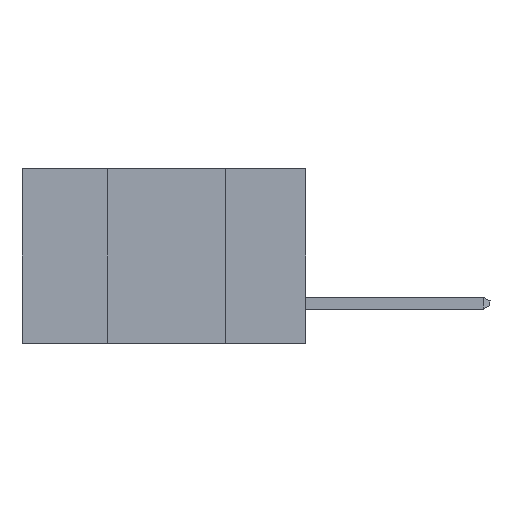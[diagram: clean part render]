
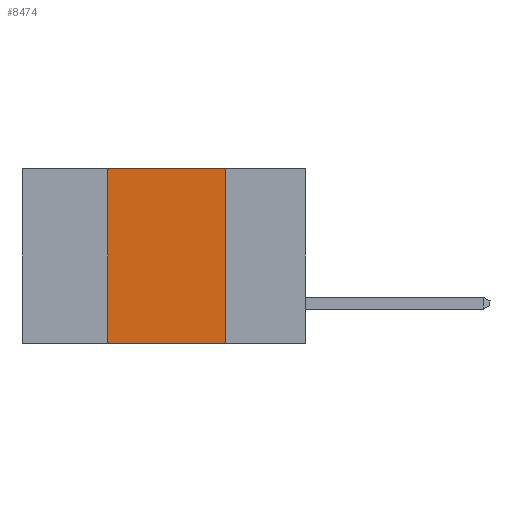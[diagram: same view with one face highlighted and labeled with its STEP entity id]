
A CAD part, left-side view. The second image highlights one B-rep face of the part: STEP entity #8474.
In plain terms, the highlighted planar face has unit normal (-1, 0, 0).
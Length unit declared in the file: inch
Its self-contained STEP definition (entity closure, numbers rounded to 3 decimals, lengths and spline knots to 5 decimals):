
#696 = CARTESIAN_POINT ( 'NONE',  ( 0., 0.42, -0.37 ) ) ;
#1284 = DIRECTION ( 'NONE',  ( 0., 0., -1. ) ) ;
#1611 = CARTESIAN_POINT ( 'NONE',  ( 0., 0.17, 0. ) ) ;
#1763 = VERTEX_POINT ( 'NONE', #1611 ) ;
#1956 = ORIENTED_EDGE ( 'NONE', *, *, #2727, .F. ) ;
#2432 = CARTESIAN_POINT ( 'NONE',  ( 0., 0.17, 0. ) ) ;
#2727 = EDGE_CURVE ( 'NONE', #1763, #9003, #4793, .T. ) ;
#2791 = LINE ( 'NONE', #11606, #6985 ) ;
#4359 = VECTOR ( 'NONE', #7075, 39.37008 ) ;
#4793 = LINE ( 'NONE', #2432, #9816 ) ;
#4835 = EDGE_CURVE ( 'NONE', #6729, #11864, #10632, .T. ) ;
#5705 = EDGE_CURVE ( 'NONE', #6729, #9003, #11874, .T. ) ;
#6604 = EDGE_CURVE ( 'NONE', #11864, #1763, #2791, .T. ) ;
#6729 = VERTEX_POINT ( 'NONE', #696 ) ;
#6985 = VECTOR ( 'NONE', #7685, 39.37008 ) ;
#7075 = DIRECTION ( 'NONE',  ( 0., -1., 0. ) ) ;
#7654 = CARTESIAN_POINT ( 'NONE',  ( 0., 0.42, 0. ) ) ;
#7685 = DIRECTION ( 'NONE',  ( 0., -1., 0. ) ) ;
#8192 = PLANE ( 'NONE',  #9894 ) ;
#8474 = ADVANCED_FACE ( 'NONE', ( #8698 ), #8192, .F. ) ;
#8698 = FACE_OUTER_BOUND ( 'NONE', #11669, .T. ) ;
#9003 = VERTEX_POINT ( 'NONE', #11576 ) ;
#9061 = CARTESIAN_POINT ( 'NONE',  ( 0., 0.6, 0. ) ) ;
#9583 = DIRECTION ( 'NONE',  ( 0., 0., 1. ) ) ;
#9636 = CARTESIAN_POINT ( 'NONE',  ( 0., 0.42, 0. ) ) ;
#9816 = VECTOR ( 'NONE', #12527, 39.37008 ) ;
#9894 = AXIS2_PLACEMENT_3D ( 'NONE', #9061, #11673, #1284 ) ;
#10091 = ORIENTED_EDGE ( 'NONE', *, *, #5705, .T. ) ;
#10632 = LINE ( 'NONE', #7654, #11869 ) ;
#11571 = ORIENTED_EDGE ( 'NONE', *, *, #6604, .F. ) ;
#11576 = CARTESIAN_POINT ( 'NONE',  ( 0., 0.17, -0.37 ) ) ;
#11606 = CARTESIAN_POINT ( 'NONE',  ( 0., 0.6, 0. ) ) ;
#11669 = EDGE_LOOP ( 'NONE', ( #1956, #11571, #11967, #10091 ) ) ;
#11673 = DIRECTION ( 'NONE',  ( 1., 0., 0. ) ) ;
#11864 = VERTEX_POINT ( 'NONE', #9636 ) ;
#11869 = VECTOR ( 'NONE', #9583, 39.37008 ) ;
#11874 = LINE ( 'NONE', #11937, #4359 ) ;
#11937 = CARTESIAN_POINT ( 'NONE',  ( 0., 0.6, -0.37 ) ) ;
#11967 = ORIENTED_EDGE ( 'NONE', *, *, #4835, .F. ) ;
#12527 = DIRECTION ( 'NONE',  ( 0., 0., -1. ) ) ;
